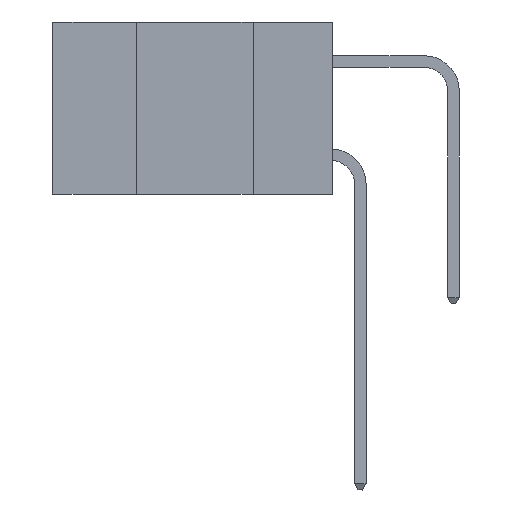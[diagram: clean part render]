
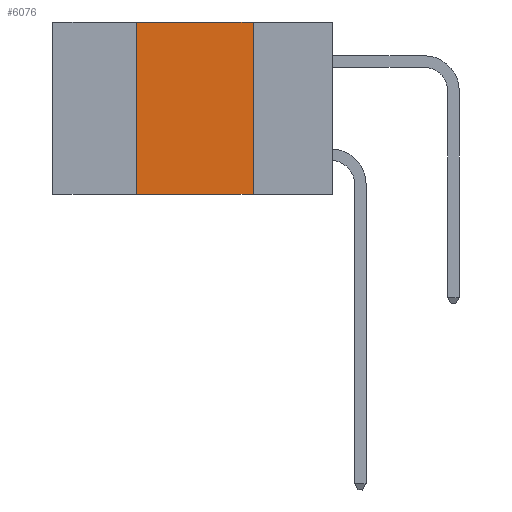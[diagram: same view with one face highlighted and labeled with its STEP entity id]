
A CAD part, left-side view. The second image highlights one B-rep face of the part: STEP entity #6076.
In plain terms, the highlighted planar face has unit normal (-1, 0, 0).
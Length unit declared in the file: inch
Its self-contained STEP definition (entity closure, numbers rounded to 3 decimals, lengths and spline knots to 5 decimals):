
#301 = CARTESIAN_POINT ( 'NONE',  ( 0., 0.6, 0. ) ) ;
#546 = CARTESIAN_POINT ( 'NONE',  ( 0., 0.17, 0. ) ) ;
#1303 = AXIS2_PLACEMENT_3D ( 'NONE', #7420, #7374, #10271 ) ;
#1418 = ORIENTED_EDGE ( 'NONE', *, *, #7658, .T. ) ;
#2267 = DIRECTION ( 'NONE',  ( 0., -1., 0. ) ) ;
#3159 = VERTEX_POINT ( 'NONE', #546 ) ;
#3209 = CARTESIAN_POINT ( 'NONE',  ( 0., 0.42, 0. ) ) ;
#3253 = EDGE_LOOP ( 'NONE', ( #4480, #8498, #8469, #1418 ) ) ;
#3747 = EDGE_CURVE ( 'NONE', #4061, #9123, #7620, .T. ) ;
#4061 = VERTEX_POINT ( 'NONE', #4218 ) ;
#4218 = CARTESIAN_POINT ( 'NONE',  ( 0., 0.42, -0.37 ) ) ;
#4480 = ORIENTED_EDGE ( 'NONE', *, *, #10111, .F. ) ;
#4857 = CARTESIAN_POINT ( 'NONE',  ( 0., 0.17, 0. ) ) ;
#4952 = VECTOR ( 'NONE', #7834, 39.37008 ) ;
#5168 = FACE_OUTER_BOUND ( 'NONE', #3253, .T. ) ;
#5969 = LINE ( 'NONE', #301, #12069 ) ;
#6076 = ADVANCED_FACE ( 'NONE', ( #5168 ), #7328, .F. ) ;
#6082 = CARTESIAN_POINT ( 'NONE',  ( 0., 0.42, 0. ) ) ;
#6764 = CARTESIAN_POINT ( 'NONE',  ( 0., 0.17, -0.37 ) ) ;
#7282 = DIRECTION ( 'NONE',  ( 0., -1., 0. ) ) ;
#7328 = PLANE ( 'NONE',  #1303 ) ;
#7374 = DIRECTION ( 'NONE',  ( 1., 0., 0. ) ) ;
#7420 = CARTESIAN_POINT ( 'NONE',  ( 0., 0.6, 0. ) ) ;
#7620 = LINE ( 'NONE', #6082, #11044 ) ;
#7658 = EDGE_CURVE ( 'NONE', #4061, #11411, #11563, .T. ) ;
#7834 = DIRECTION ( 'NONE',  ( 0., 0., -1. ) ) ;
#8469 = ORIENTED_EDGE ( 'NONE', *, *, #3747, .F. ) ;
#8498 = ORIENTED_EDGE ( 'NONE', *, *, #11530, .F. ) ;
#9123 = VERTEX_POINT ( 'NONE', #3209 ) ;
#9454 = DIRECTION ( 'NONE',  ( 0., 0., 1. ) ) ;
#10009 = LINE ( 'NONE', #4857, #4952 ) ;
#10111 = EDGE_CURVE ( 'NONE', #3159, #11411, #10009, .T. ) ;
#10185 = CARTESIAN_POINT ( 'NONE',  ( 0., 0.6, -0.37 ) ) ;
#10271 = DIRECTION ( 'NONE',  ( 0., 0., -1. ) ) ;
#11044 = VECTOR ( 'NONE', #9454, 39.37008 ) ;
#11108 = VECTOR ( 'NONE', #7282, 39.37008 ) ;
#11411 = VERTEX_POINT ( 'NONE', #6764 ) ;
#11530 = EDGE_CURVE ( 'NONE', #9123, #3159, #5969, .T. ) ;
#11563 = LINE ( 'NONE', #10185, #11108 ) ;
#12069 = VECTOR ( 'NONE', #2267, 39.37008 ) ;
